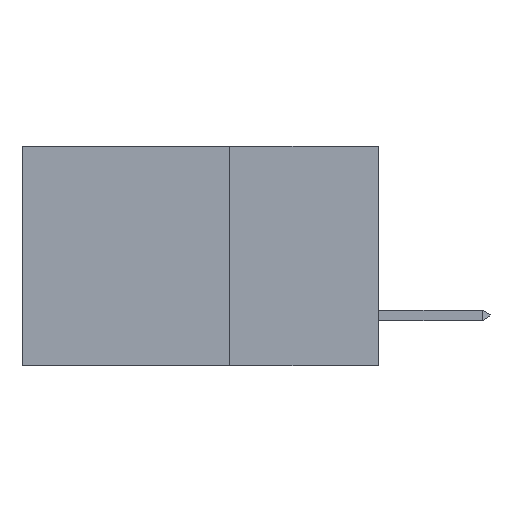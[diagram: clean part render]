
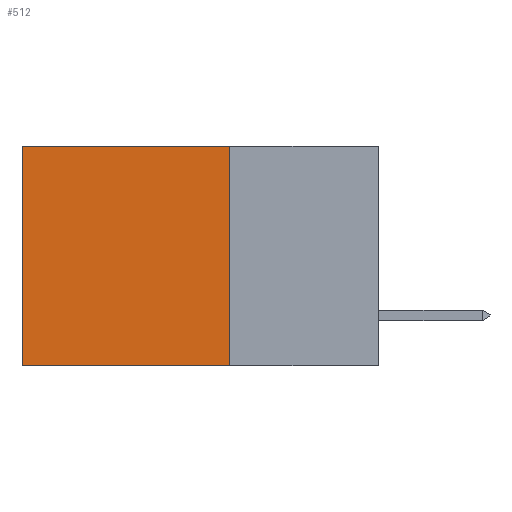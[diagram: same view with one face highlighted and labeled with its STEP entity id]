
A CAD part, left-side view. The second image highlights one B-rep face of the part: STEP entity #512.
In plain terms, the highlighted planar face has unit normal (-1, 0, 0).
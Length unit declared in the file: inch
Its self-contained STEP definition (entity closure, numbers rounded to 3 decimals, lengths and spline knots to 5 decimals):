
#193 = VERTEX_POINT ( 'NONE', #2559 ) ;
#512 = ADVANCED_FACE ( 'NONE', ( #7985 ), #2167, .F. ) ;
#1654 = VECTOR ( 'NONE', #13145, 39.37008 ) ;
#2089 = VECTOR ( 'NONE', #11437, 39.37008 ) ;
#2167 = PLANE ( 'NONE',  #10562 ) ;
#2476 = ORIENTED_EDGE ( 'NONE', *, *, #12509, .T. ) ;
#2559 = CARTESIAN_POINT ( 'NONE',  ( 0.2615, 0.25, -0.37 ) ) ;
#2767 = ORIENTED_EDGE ( 'NONE', *, *, #12579, .F. ) ;
#2890 = VECTOR ( 'NONE', #9892, 39.37008 ) ;
#3092 = EDGE_CURVE ( 'NONE', #12310, #11357, #3353, .T. ) ;
#3095 = DIRECTION ( 'NONE',  ( 1., 0., 0. ) ) ;
#3353 = LINE ( 'NONE', #8016, #2890 ) ;
#5572 = CARTESIAN_POINT ( 'NONE',  ( 0.2615, 0.25, -0.37 ) ) ;
#6129 = LINE ( 'NONE', #8350, #1654 ) ;
#7048 = CARTESIAN_POINT ( 'NONE',  ( 0.2615, 0.25, -0.37 ) ) ;
#7244 = ORIENTED_EDGE ( 'NONE', *, *, #3092, .T. ) ;
#7343 = LINE ( 'NONE', #7048, #9271 ) ;
#7768 = DIRECTION ( 'NONE',  ( 0., 0., -1. ) ) ;
#7985 = FACE_OUTER_BOUND ( 'NONE', #8324, .T. ) ;
#8016 = CARTESIAN_POINT ( 'NONE',  ( 0.2615, 0.25, 0. ) ) ;
#8324 = EDGE_LOOP ( 'NONE', ( #2476, #15212, #2767, #7244 ) ) ;
#8350 = CARTESIAN_POINT ( 'NONE',  ( 0.2615, 0.6, -0.37 ) ) ;
#9271 = VECTOR ( 'NONE', #14146, 39.37008 ) ;
#9505 = EDGE_CURVE ( 'NONE', #193, #14115, #12900, .T. ) ;
#9892 = DIRECTION ( 'NONE',  ( 0., 1., 0. ) ) ;
#10562 = AXIS2_PLACEMENT_3D ( 'NONE', #13648, #3095, #7768 ) ;
#11357 = VERTEX_POINT ( 'NONE', #14302 ) ;
#11437 = DIRECTION ( 'NONE',  ( 0., 1., 0. ) ) ;
#12237 = CARTESIAN_POINT ( 'NONE',  ( 0.2615, 0.25, 0. ) ) ;
#12310 = VERTEX_POINT ( 'NONE', #12237 ) ;
#12509 = EDGE_CURVE ( 'NONE', #11357, #14115, #6129, .T. ) ;
#12579 = EDGE_CURVE ( 'NONE', #12310, #193, #7343, .T. ) ;
#12900 = LINE ( 'NONE', #5572, #2089 ) ;
#13145 = DIRECTION ( 'NONE',  ( 0., 0., -1. ) ) ;
#13648 = CARTESIAN_POINT ( 'NONE',  ( 0.2615, 0.25, -0.37 ) ) ;
#14115 = VERTEX_POINT ( 'NONE', #14916 ) ;
#14146 = DIRECTION ( 'NONE',  ( 0., 0., -1. ) ) ;
#14302 = CARTESIAN_POINT ( 'NONE',  ( 0.2615, 0.6, 0. ) ) ;
#14916 = CARTESIAN_POINT ( 'NONE',  ( 0.2615, 0.6, -0.37 ) ) ;
#15212 = ORIENTED_EDGE ( 'NONE', *, *, #9505, .F. ) ;
